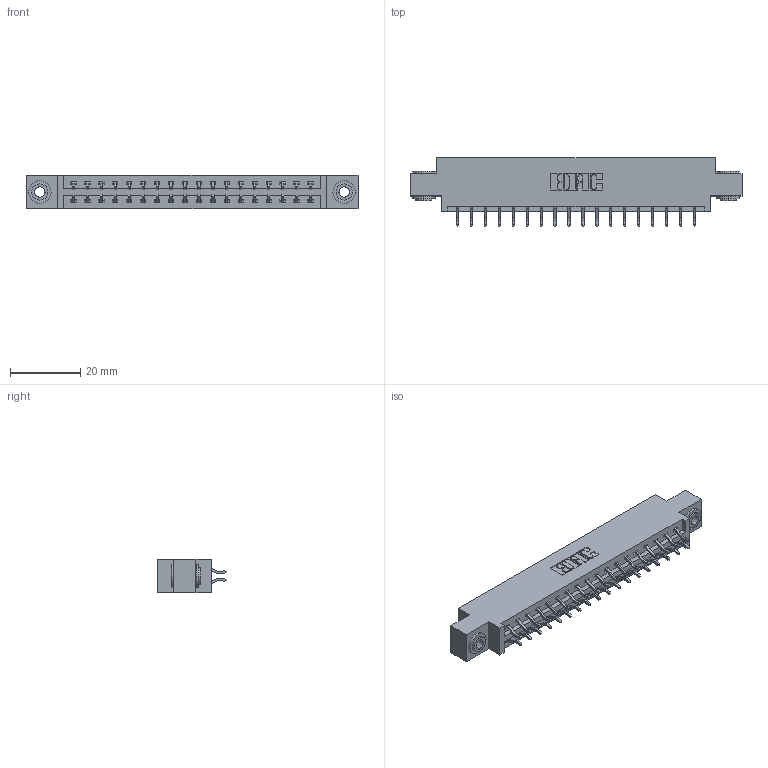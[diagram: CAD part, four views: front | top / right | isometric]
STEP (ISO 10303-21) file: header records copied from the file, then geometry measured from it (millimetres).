
FILE_DESCRIPTION (( 'STEP AP203' ), '1' );
FILE_NAME ('387-036-556-803.STEP', '2018-09-19T01:18:48', ( '' ), ( '' ), 'SwSTEP 2.0', 'SolidWorks 2016', '' );
FILE_SCHEMA (( 'CONFIG_CONTROL_DESIGN' ));
Length unit declared in the file: inch
Products named in the file (4): 337 Part_0.170 Offset - 0.156 Dia-TH; 345-292-001_556 Tail; 345-250-002_345-250-002-102; 387-036-556-803
Assembly tree (39 placements, depth 2):
  387-036-556-803
    337 Part_0.170 Offset - 0.156 Dia-TH
    345-292-001_556 Tail  x36
    345-250-002_345-250-002-102  x2
Bounding box: 94.34 x 19.57 x 9.4 mm (x, y, z)
Volume: 9522.8 mm3; surface area: 10826.7 mm2
Topology: 39 solids, 39 shells, 2316 faces, 6843 edges, 4510 vertices
Faces by surface type: plane 1596, cylinder 712, cone 8
Entity records: 18062 total; most frequent: CARTESIAN_POINT 3053, ORIENTED_EDGE 2970, DIRECTION 2663, EDGE_CURVE 1485, LINE 1325, VECTOR 1325, VERTEX_POINT 986, AXIS2_PLACEMENT_3D 669
